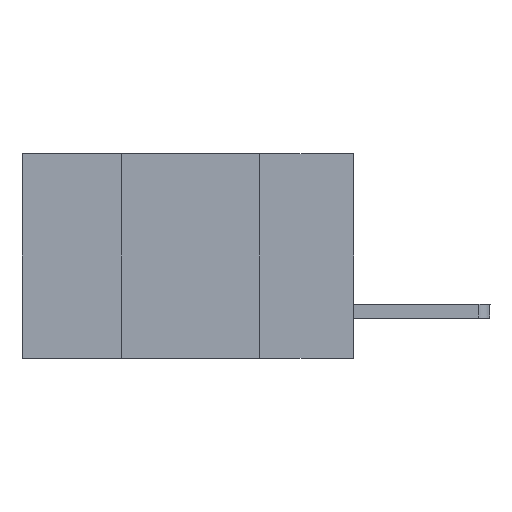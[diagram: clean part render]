
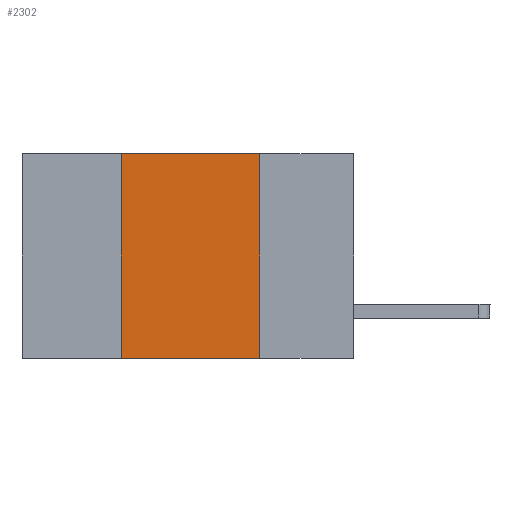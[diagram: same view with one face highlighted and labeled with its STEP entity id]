
A CAD part, left-side view. The second image highlights one B-rep face of the part: STEP entity #2302.
In plain terms, the highlighted planar face has unit normal (-1, 0, 0).
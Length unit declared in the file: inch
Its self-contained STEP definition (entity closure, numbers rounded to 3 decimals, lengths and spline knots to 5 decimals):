
#37 = AXIS2_PLACEMENT_3D ( 'NONE', #6373, #3833, #5480 ) ;
#220 = ORIENTED_EDGE ( 'NONE', *, *, #1867, .F. ) ;
#382 = VERTEX_POINT ( 'NONE', #4394 ) ;
#1069 = VERTEX_POINT ( 'NONE', #7189 ) ;
#1074 = LINE ( 'NONE', #1747, #7427 ) ;
#1275 = EDGE_CURVE ( 'NONE', #7908, #5806, #8377, .T. ) ;
#1309 = ORIENTED_EDGE ( 'NONE', *, *, #1275, .T. ) ;
#1712 = DIRECTION ( 'NONE',  ( 0., 0., 1. ) ) ;
#1747 = CARTESIAN_POINT ( 'NONE',  ( 0., 0.42, 0. ) ) ;
#1867 = EDGE_CURVE ( 'NONE', #1069, #5806, #8366, .T. ) ;
#1910 = DIRECTION ( 'NONE',  ( 0., -1., 0. ) ) ;
#2302 = ADVANCED_FACE ( 'NONE', ( #4189 ), #4636, .F. ) ;
#2454 = DIRECTION ( 'NONE',  ( 0., 0., -1. ) ) ;
#2573 = ORIENTED_EDGE ( 'NONE', *, *, #6621, .F. ) ;
#2862 = ORIENTED_EDGE ( 'NONE', *, *, #8632, .F. ) ;
#3833 = DIRECTION ( 'NONE',  ( 1., 0., 0. ) ) ;
#3926 = LINE ( 'NONE', #10431, #4451 ) ;
#4189 = FACE_OUTER_BOUND ( 'NONE', #5228, .T. ) ;
#4355 = CARTESIAN_POINT ( 'NONE',  ( 0., 0.6, -0.37 ) ) ;
#4394 = CARTESIAN_POINT ( 'NONE',  ( 0., 0.42, 0. ) ) ;
#4451 = VECTOR ( 'NONE', #6372, 39.37008 ) ;
#4608 = CARTESIAN_POINT ( 'NONE',  ( 0., 0.42, -0.37 ) ) ;
#4636 = PLANE ( 'NONE',  #37 ) ;
#4879 = VECTOR ( 'NONE', #2454, 39.37008 ) ;
#5228 = EDGE_LOOP ( 'NONE', ( #220, #2862, #2573, #1309 ) ) ;
#5480 = DIRECTION ( 'NONE',  ( 0., 0., -1. ) ) ;
#5806 = VERTEX_POINT ( 'NONE', #7987 ) ;
#5947 = VECTOR ( 'NONE', #1910, 39.37008 ) ;
#6372 = DIRECTION ( 'NONE',  ( 0., -1., 0. ) ) ;
#6373 = CARTESIAN_POINT ( 'NONE',  ( 0., 0.6, 0. ) ) ;
#6621 = EDGE_CURVE ( 'NONE', #7908, #382, #1074, .T. ) ;
#7189 = CARTESIAN_POINT ( 'NONE',  ( 0., 0.17, 0. ) ) ;
#7427 = VECTOR ( 'NONE', #1712, 39.37008 ) ;
#7486 = CARTESIAN_POINT ( 'NONE',  ( 0., 0.17, 0. ) ) ;
#7908 = VERTEX_POINT ( 'NONE', #4608 ) ;
#7987 = CARTESIAN_POINT ( 'NONE',  ( 0., 0.17, -0.37 ) ) ;
#8366 = LINE ( 'NONE', #7486, #4879 ) ;
#8377 = LINE ( 'NONE', #4355, #5947 ) ;
#8632 = EDGE_CURVE ( 'NONE', #382, #1069, #3926, .T. ) ;
#10431 = CARTESIAN_POINT ( 'NONE',  ( 0., 0.6, 0. ) ) ;
